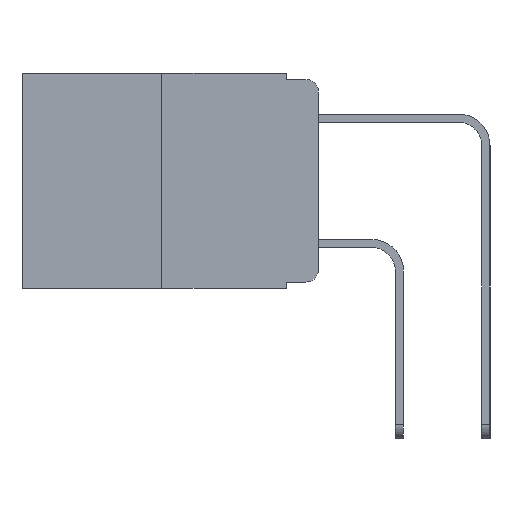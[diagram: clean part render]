
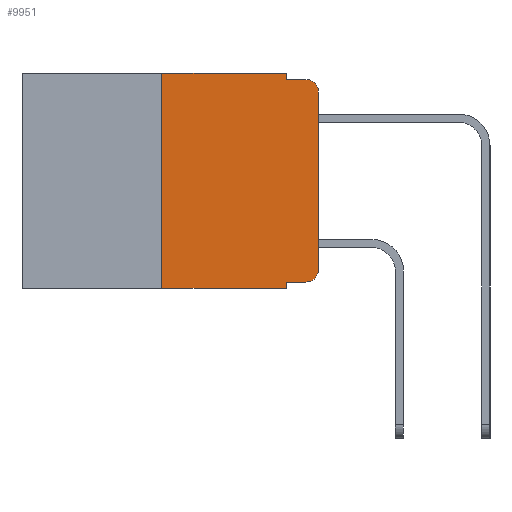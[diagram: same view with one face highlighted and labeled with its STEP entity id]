
A CAD part, left-side view. The second image highlights one B-rep face of the part: STEP entity #9951.
In plain terms, the highlighted planar face has unit normal (-1, 0, 0).
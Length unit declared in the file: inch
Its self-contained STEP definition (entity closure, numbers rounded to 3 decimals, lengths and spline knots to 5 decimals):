
#434 = DIRECTION ( 'NONE',  ( 0., 0., -1. ) ) ;
#757 = LINE ( 'NONE', #2190, #20520 ) ;
#816 = EDGE_CURVE ( 'NONE', #17173, #14545, #12259, .T. ) ;
#1014 = ORIENTED_EDGE ( 'NONE', *, *, #18856, .T. ) ;
#1174 = DIRECTION ( 'NONE',  ( 0., -1., 0. ) ) ;
#1260 = CARTESIAN_POINT ( 'NONE',  ( 0., 0.473, 0. ) ) ;
#1651 = EDGE_CURVE ( 'NONE', #4352, #8686, #21774, .T. ) ;
#2190 = CARTESIAN_POINT ( 'NONE',  ( 0., 0.051, -0.01 ) ) ;
#2422 = VERTEX_POINT ( 'NONE', #22352 ) ;
#2506 = CARTESIAN_POINT ( 'NONE',  ( 0., 0.051, 0. ) ) ;
#2980 = DIRECTION ( 'NONE',  ( 0., 0., -1. ) ) ;
#3390 = DIRECTION ( 'NONE',  ( -1., 0., 0. ) ) ;
#3740 = CARTESIAN_POINT ( 'NONE',  ( 0., 0.25, -0.343 ) ) ;
#4028 = DIRECTION ( 'NONE',  ( 0., -1., 0. ) ) ;
#4352 = VERTEX_POINT ( 'NONE', #3740 ) ;
#4468 = DIRECTION ( 'NONE',  ( 0., 0., -1. ) ) ;
#5456 = CARTESIAN_POINT ( 'NONE',  ( 0., 0.051, -0.01 ) ) ;
#5578 = EDGE_CURVE ( 'NONE', #18578, #17198, #24456, .T. ) ;
#5582 = ORIENTED_EDGE ( 'NONE', *, *, #21363, .F. ) ;
#6514 = ORIENTED_EDGE ( 'NONE', *, *, #17152, .T. ) ;
#6822 = EDGE_CURVE ( 'NONE', #4352, #11372, #20407, .T. ) ;
#7084 = LINE ( 'NONE', #1260, #16671 ) ;
#7165 = CARTESIAN_POINT ( 'NONE',  ( 0., 0.02, -0.01 ) ) ;
#7670 = CARTESIAN_POINT ( 'NONE',  ( 0., 0.051, -0.333 ) ) ;
#7820 = DIRECTION ( 'NONE',  ( -1., 0., 0. ) ) ;
#8686 = VERTEX_POINT ( 'NONE', #22411 ) ;
#8722 = ORIENTED_EDGE ( 'NONE', *, *, #816, .T. ) ;
#9321 = VECTOR ( 'NONE', #22651, 39.37008 ) ;
#9951 = ADVANCED_FACE ( 'NONE', ( #10021 ), #18595, .F. ) ;
#10021 = FACE_OUTER_BOUND ( 'NONE', #17020, .T. ) ;
#10456 = LINE ( 'NONE', #2506, #12116 ) ;
#10677 = CARTESIAN_POINT ( 'NONE',  ( 0., 0.051, -0.343 ) ) ;
#11132 = ORIENTED_EDGE ( 'NONE', *, *, #22496, .F. ) ;
#11149 = DIRECTION ( 'NONE',  ( 0., 0., -1. ) ) ;
#11372 = VERTEX_POINT ( 'NONE', #10677 ) ;
#11736 = ORIENTED_EDGE ( 'NONE', *, *, #13424, .F. ) ;
#11970 = VECTOR ( 'NONE', #17691, 39.37008 ) ;
#12116 = VECTOR ( 'NONE', #4468, 39.37008 ) ;
#12259 = CIRCLE ( 'NONE', #17911, 0.02 ) ;
#12332 = ORIENTED_EDGE ( 'NONE', *, *, #5578, .F. ) ;
#12727 = CARTESIAN_POINT ( 'NONE',  ( 0., 0.051, 0. ) ) ;
#13424 = EDGE_CURVE ( 'NONE', #17198, #15604, #757, .T. ) ;
#14328 = AXIS2_PLACEMENT_3D ( 'NONE', #15021, #3390, #16879 ) ;
#14545 = VERTEX_POINT ( 'NONE', #24385 ) ;
#14578 = CARTESIAN_POINT ( 'NONE',  ( 0., 0., 0. ) ) ;
#14715 = AXIS2_PLACEMENT_3D ( 'NONE', #20441, #22248, #11149 ) ;
#15021 = CARTESIAN_POINT ( 'NONE',  ( 0., 0.02, -0.03 ) ) ;
#15604 = VERTEX_POINT ( 'NONE', #7165 ) ;
#16117 = VECTOR ( 'NONE', #4028, 39.37008 ) ;
#16260 = CIRCLE ( 'NONE', #14328, 0.02 ) ;
#16455 = DIRECTION ( 'NONE',  ( 0., 0., 1. ) ) ;
#16671 = VECTOR ( 'NONE', #1174, 39.37008 ) ;
#16879 = DIRECTION ( 'NONE',  ( 0., 0., -1. ) ) ;
#16884 = CARTESIAN_POINT ( 'NONE',  ( 0., 0.02, -0.313 ) ) ;
#17020 = EDGE_LOOP ( 'NONE', ( #23551, #6514, #11736, #12332, #5582, #21303, #19891, #11132, #1014, #8722 ) ) ;
#17152 = EDGE_CURVE ( 'NONE', #21225, #15604, #16260, .T. ) ;
#17173 = VERTEX_POINT ( 'NONE', #20584 ) ;
#17198 = VERTEX_POINT ( 'NONE', #5456 ) ;
#17485 = CARTESIAN_POINT ( 'NONE',  ( 0., 0.473, -0.343 ) ) ;
#17587 = DIRECTION ( 'NONE',  ( 0., -1., 0. ) ) ;
#17691 = DIRECTION ( 'NONE',  ( 0., 0., 1. ) ) ;
#17911 = AXIS2_PLACEMENT_3D ( 'NONE', #16884, #7820, #434 ) ;
#18265 = CARTESIAN_POINT ( 'NONE',  ( 0., 0., -0.03 ) ) ;
#18578 = VERTEX_POINT ( 'NONE', #20203 ) ;
#18595 = PLANE ( 'NONE',  #14715 ) ;
#18856 = EDGE_CURVE ( 'NONE', #2422, #17173, #19892, .T. ) ;
#19005 = CARTESIAN_POINT ( 'NONE',  ( 0., 0.25, 0. ) ) ;
#19058 = VECTOR ( 'NONE', #2980, 39.37008 ) ;
#19891 = ORIENTED_EDGE ( 'NONE', *, *, #6822, .T. ) ;
#19892 = LINE ( 'NONE', #7670, #9321 ) ;
#20203 = CARTESIAN_POINT ( 'NONE',  ( 0., 0.051, 0. ) ) ;
#20407 = LINE ( 'NONE', #17485, #16117 ) ;
#20441 = CARTESIAN_POINT ( 'NONE',  ( 0., 0.473, 0. ) ) ;
#20520 = VECTOR ( 'NONE', #17587, 39.37008 ) ;
#20584 = CARTESIAN_POINT ( 'NONE',  ( 0., 0.02, -0.333 ) ) ;
#21225 = VERTEX_POINT ( 'NONE', #18265 ) ;
#21303 = ORIENTED_EDGE ( 'NONE', *, *, #1651, .F. ) ;
#21363 = EDGE_CURVE ( 'NONE', #8686, #18578, #7084, .T. ) ;
#21774 = LINE ( 'NONE', #19005, #11970 ) ;
#22045 = EDGE_CURVE ( 'NONE', #14545, #21225, #23499, .T. ) ;
#22248 = DIRECTION ( 'NONE',  ( 1., 0., 0. ) ) ;
#22352 = CARTESIAN_POINT ( 'NONE',  ( 0., 0.051, -0.333 ) ) ;
#22411 = CARTESIAN_POINT ( 'NONE',  ( 0., 0.25, 0. ) ) ;
#22496 = EDGE_CURVE ( 'NONE', #2422, #11372, #10456, .T. ) ;
#22651 = DIRECTION ( 'NONE',  ( 0., -1., 0. ) ) ;
#22930 = VECTOR ( 'NONE', #16455, 39.37008 ) ;
#23499 = LINE ( 'NONE', #14578, #22930 ) ;
#23551 = ORIENTED_EDGE ( 'NONE', *, *, #22045, .T. ) ;
#24385 = CARTESIAN_POINT ( 'NONE',  ( 0., 0., -0.313 ) ) ;
#24456 = LINE ( 'NONE', #12727, #19058 ) ;
